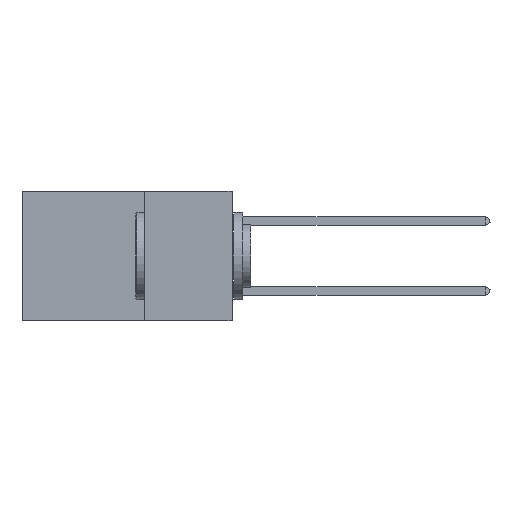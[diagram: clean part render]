
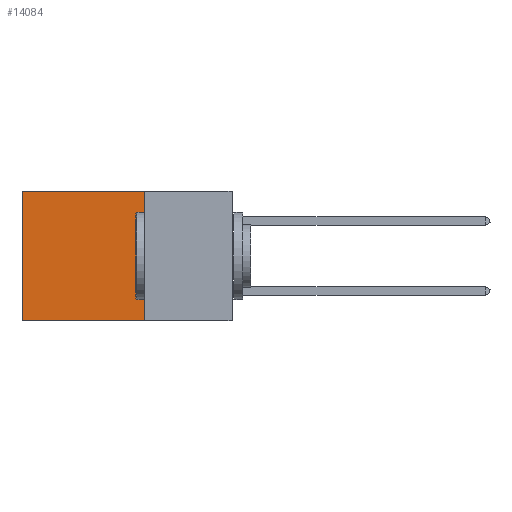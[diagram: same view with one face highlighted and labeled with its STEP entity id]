
A CAD part, left-side view. The second image highlights one B-rep face of the part: STEP entity #14084.
In plain terms, the highlighted planar face has unit normal (-1, 0, 0).
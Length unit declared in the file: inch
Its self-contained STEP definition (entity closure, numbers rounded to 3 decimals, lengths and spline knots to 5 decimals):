
#402 = VECTOR ( 'NONE', #21228, 39.37008 ) ;
#607 = VECTOR ( 'NONE', #23468, 39.37008 ) ;
#706 = ORIENTED_EDGE ( 'NONE', *, *, #9275, .F. ) ;
#1053 = DIRECTION ( 'NONE',  ( 0., 1., 0. ) ) ;
#1354 = LINE ( 'NONE', #12871, #402 ) ;
#1538 = CARTESIAN_POINT ( 'NONE',  ( 0.2875, 0.6, 0. ) ) ;
#2167 = FACE_OUTER_BOUND ( 'NONE', #2182, .T. ) ;
#2182 = EDGE_LOOP ( 'NONE', ( #8392, #10880, #706, #15198 ) ) ;
#2969 = CARTESIAN_POINT ( 'NONE',  ( 0.2875, 0.25, 0. ) ) ;
#3889 = LINE ( 'NONE', #23758, #25426 ) ;
#5701 = AXIS2_PLACEMENT_3D ( 'NONE', #24316, #27103, #10963 ) ;
#6133 = CARTESIAN_POINT ( 'NONE',  ( 0.2875, 0.6, -0.37 ) ) ;
#6287 = VERTEX_POINT ( 'NONE', #2969 ) ;
#8392 = ORIENTED_EDGE ( 'NONE', *, *, #30630, .T. ) ;
#9275 = EDGE_CURVE ( 'NONE', #6287, #17451, #15932, .T. ) ;
#10880 = ORIENTED_EDGE ( 'NONE', *, *, #28027, .F. ) ;
#10963 = DIRECTION ( 'NONE',  ( 0., 0., -1. ) ) ;
#11270 = CARTESIAN_POINT ( 'NONE',  ( 0.2875, 0.25, -0.37 ) ) ;
#12487 = CARTESIAN_POINT ( 'NONE',  ( 0.2875, 0.25, 0. ) ) ;
#12871 = CARTESIAN_POINT ( 'NONE',  ( 0.2875, 0.25, 0. ) ) ;
#14084 = ADVANCED_FACE ( 'NONE', ( #2167 ), #18802, .F. ) ;
#15198 = ORIENTED_EDGE ( 'NONE', *, *, #15984, .T. ) ;
#15932 = LINE ( 'NONE', #12487, #607 ) ;
#15984 = EDGE_CURVE ( 'NONE', #6287, #32146, #1354, .T. ) ;
#17451 = VERTEX_POINT ( 'NONE', #11270 ) ;
#18802 = PLANE ( 'NONE',  #5701 ) ;
#21228 = DIRECTION ( 'NONE',  ( 0., 1., 0. ) ) ;
#23468 = DIRECTION ( 'NONE',  ( 0., 0., -1. ) ) ;
#23758 = CARTESIAN_POINT ( 'NONE',  ( 0.2875, 0.6, 0. ) ) ;
#24316 = CARTESIAN_POINT ( 'NONE',  ( 0.2875, 0.25, 0. ) ) ;
#25426 = VECTOR ( 'NONE', #26547, 39.37008 ) ;
#26547 = DIRECTION ( 'NONE',  ( 0., 0., -1. ) ) ;
#27103 = DIRECTION ( 'NONE',  ( 1., 0., 0. ) ) ;
#27386 = VECTOR ( 'NONE', #1053, 39.37008 ) ;
#28027 = EDGE_CURVE ( 'NONE', #17451, #30435, #28235, .T. ) ;
#28235 = LINE ( 'NONE', #34566, #27386 ) ;
#30435 = VERTEX_POINT ( 'NONE', #6133 ) ;
#30630 = EDGE_CURVE ( 'NONE', #32146, #30435, #3889, .T. ) ;
#32146 = VERTEX_POINT ( 'NONE', #1538 ) ;
#34566 = CARTESIAN_POINT ( 'NONE',  ( 0.2875, 0.25, -0.37 ) ) ;
